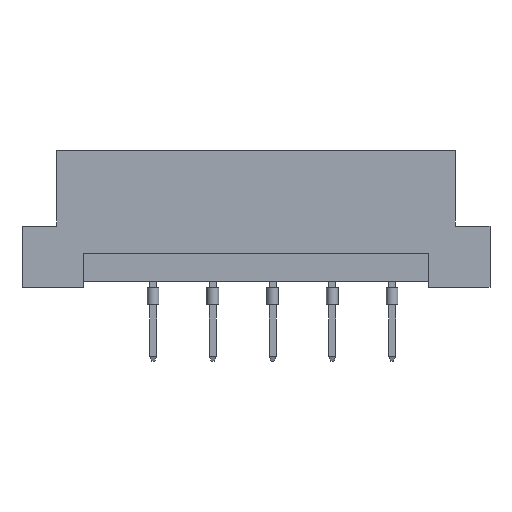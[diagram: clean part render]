
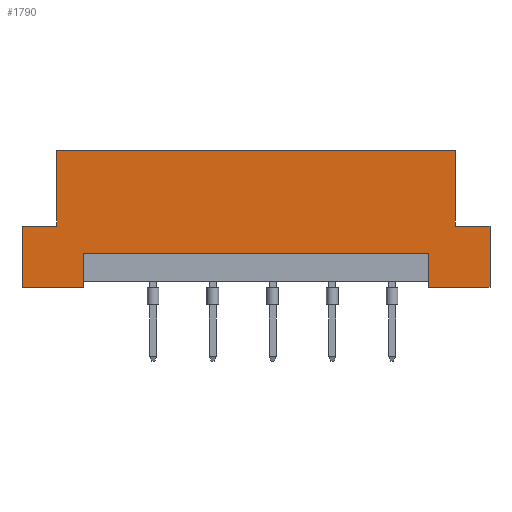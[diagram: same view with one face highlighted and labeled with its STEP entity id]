
A CAD part, front view. The second image highlights one B-rep face of the part: STEP entity #1790.
In plain terms, the highlighted planar face has unit normal (0, -1, 0).
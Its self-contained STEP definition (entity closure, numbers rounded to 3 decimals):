
#27 = CARTESIAN_POINT ( 'NONE',  ( -19.9, 0., 0. ) ) ;
#68 = LINE ( 'NONE', #2742, #5200 ) ;
#84 = CARTESIAN_POINT ( 'NONE',  ( -19.9, 0., 0. ) ) ;
#113 = LINE ( 'NONE', #6274, #5737 ) ;
#240 = VECTOR ( 'NONE', #1195, 1000. ) ;
#300 = VECTOR ( 'NONE', #1503, 1000. ) ;
#323 = ORIENTED_EDGE ( 'NONE', *, *, #650, .F. ) ;
#354 = DIRECTION ( 'NONE',  ( 0., 0., 1. ) ) ;
#372 = DIRECTION ( 'NONE',  ( 1., 0., 0. ) ) ;
#427 = ORIENTED_EDGE ( 'NONE', *, *, #1605, .F. ) ;
#447 = LINE ( 'NONE', #6684, #300 ) ;
#557 = DIRECTION ( 'NONE',  ( 1., 0., 0. ) ) ;
#596 = DIRECTION ( 'NONE',  ( 0., 0., -1. ) ) ;
#650 = EDGE_CURVE ( 'NONE', #3738, #4170, #4349, .T. ) ;
#774 = CARTESIAN_POINT ( 'NONE',  ( -16.94, 0., 5.2 ) ) ;
#821 = EDGE_CURVE ( 'NONE', #1131, #5283, #1346, .T. ) ;
#930 = CARTESIAN_POINT ( 'NONE',  ( 19.9, 0., 0. ) ) ;
#932 = CARTESIAN_POINT ( 'NONE',  ( -14.69, 0., 0. ) ) ;
#944 = CARTESIAN_POINT ( 'NONE',  ( 16.94, 0., 11.6 ) ) ;
#1004 = VERTEX_POINT ( 'NONE', #930 ) ;
#1118 = EDGE_CURVE ( 'NONE', #2424, #4580, #1618, .T. ) ;
#1131 = VERTEX_POINT ( 'NONE', #5353 ) ;
#1138 = EDGE_CURVE ( 'NONE', #5283, #4580, #113, .T. ) ;
#1169 = VECTOR ( 'NONE', #4728, 1000. ) ;
#1195 = DIRECTION ( 'NONE',  ( 0., 0., -1. ) ) ;
#1198 = VERTEX_POINT ( 'NONE', #2931 ) ;
#1230 = LINE ( 'NONE', #4291, #240 ) ;
#1299 = DIRECTION ( 'NONE',  ( 0., 0., 1. ) ) ;
#1346 = LINE ( 'NONE', #774, #3846 ) ;
#1361 = LINE ( 'NONE', #5511, #3336 ) ;
#1373 = VERTEX_POINT ( 'NONE', #1498 ) ;
#1493 = VECTOR ( 'NONE', #1299, 1000. ) ;
#1498 = CARTESIAN_POINT ( 'NONE',  ( 14.69, 0., 2.9 ) ) ;
#1503 = DIRECTION ( 'NONE',  ( -1., 0., 0. ) ) ;
#1559 = ORIENTED_EDGE ( 'NONE', *, *, #1784, .F. ) ;
#1605 = EDGE_CURVE ( 'NONE', #4170, #4579, #4368, .T. ) ;
#1618 = LINE ( 'NONE', #1654, #5959 ) ;
#1622 = LINE ( 'NONE', #5387, #6400 ) ;
#1654 = CARTESIAN_POINT ( 'NONE',  ( 16.94, 0., 5.2 ) ) ;
#1709 = ORIENTED_EDGE ( 'NONE', *, *, #3862, .T. ) ;
#1728 = CARTESIAN_POINT ( 'NONE',  ( -16.94, 0., 11.6 ) ) ;
#1729 = EDGE_CURVE ( 'NONE', #2424, #1198, #1361, .T. ) ;
#1784 = EDGE_CURVE ( 'NONE', #1198, #1004, #3977, .T. ) ;
#1790 = ADVANCED_FACE ( 'NONE', ( #2953 ), #4045, .F. ) ;
#2059 = EDGE_LOOP ( 'NONE', ( #2166, #1709, #3036, #1559, #6204, #4884, #3161, #4533, #6317, #427, #323, #4740 ) ) ;
#2166 = ORIENTED_EDGE ( 'NONE', *, *, #5589, .F. ) ;
#2204 = DIRECTION ( 'NONE',  ( 1., 0., 0. ) ) ;
#2424 = VERTEX_POINT ( 'NONE', #6031 ) ;
#2653 = LINE ( 'NONE', #3076, #1169 ) ;
#2742 = CARTESIAN_POINT ( 'NONE',  ( -19.9, 0., 5.2 ) ) ;
#2870 = VERTEX_POINT ( 'NONE', #3594 ) ;
#2931 = CARTESIAN_POINT ( 'NONE',  ( 19.9, 0., 5.2 ) ) ;
#2953 = FACE_OUTER_BOUND ( 'NONE', #2059, .T. ) ;
#2981 = CARTESIAN_POINT ( 'NONE',  ( -19.9, 0., 11.6 ) ) ;
#3013 = EDGE_CURVE ( 'NONE', #2870, #3738, #1230, .T. ) ;
#3036 = ORIENTED_EDGE ( 'NONE', *, *, #4673, .F. ) ;
#3076 = CARTESIAN_POINT ( 'NONE',  ( -19.9, 0., 0. ) ) ;
#3161 = ORIENTED_EDGE ( 'NONE', *, *, #1138, .F. ) ;
#3336 = VECTOR ( 'NONE', #372, 1000. ) ;
#3463 = CARTESIAN_POINT ( 'NONE',  ( -19.9, 0., 5.2 ) ) ;
#3494 = DIRECTION ( 'NONE',  ( 0., 0., -1. ) ) ;
#3594 = CARTESIAN_POINT ( 'NONE',  ( -14.69, 0., 2.9 ) ) ;
#3660 = AXIS2_PLACEMENT_3D ( 'NONE', #2981, #4500, #6120 ) ;
#3738 = VERTEX_POINT ( 'NONE', #932 ) ;
#3751 = DIRECTION ( 'NONE',  ( 0., 0., 1. ) ) ;
#3846 = VECTOR ( 'NONE', #354, 1000. ) ;
#3862 = EDGE_CURVE ( 'NONE', #1373, #5313, #1622, .T. ) ;
#3977 = LINE ( 'NONE', #5002, #6389 ) ;
#4045 = PLANE ( 'NONE',  #3660 ) ;
#4170 = VERTEX_POINT ( 'NONE', #27 ) ;
#4291 = CARTESIAN_POINT ( 'NONE',  ( -14.69, 0., 0.5 ) ) ;
#4349 = LINE ( 'NONE', #84, #5578 ) ;
#4368 = LINE ( 'NONE', #5410, #1493 ) ;
#4500 = DIRECTION ( 'NONE',  ( 0., 1., 0. ) ) ;
#4533 = ORIENTED_EDGE ( 'NONE', *, *, #821, .F. ) ;
#4579 = VERTEX_POINT ( 'NONE', #3463 ) ;
#4580 = VERTEX_POINT ( 'NONE', #944 ) ;
#4673 = EDGE_CURVE ( 'NONE', #1004, #5313, #2653, .T. ) ;
#4728 = DIRECTION ( 'NONE',  ( -1., 0., 0. ) ) ;
#4740 = ORIENTED_EDGE ( 'NONE', *, *, #3013, .F. ) ;
#4884 = ORIENTED_EDGE ( 'NONE', *, *, #1118, .T. ) ;
#5002 = CARTESIAN_POINT ( 'NONE',  ( 19.9, 0., 0. ) ) ;
#5200 = VECTOR ( 'NONE', #557, 1000. ) ;
#5228 = DIRECTION ( 'NONE',  ( -1., 0., 0. ) ) ;
#5283 = VERTEX_POINT ( 'NONE', #1728 ) ;
#5313 = VERTEX_POINT ( 'NONE', #6518 ) ;
#5353 = CARTESIAN_POINT ( 'NONE',  ( -16.94, 0., 5.2 ) ) ;
#5387 = CARTESIAN_POINT ( 'NONE',  ( 14.69, 0., 0.5 ) ) ;
#5410 = CARTESIAN_POINT ( 'NONE',  ( -19.9, 0., 0. ) ) ;
#5511 = CARTESIAN_POINT ( 'NONE',  ( 19.9, 0., 5.2 ) ) ;
#5578 = VECTOR ( 'NONE', #5228, 1000. ) ;
#5589 = EDGE_CURVE ( 'NONE', #1373, #2870, #447, .T. ) ;
#5737 = VECTOR ( 'NONE', #2204, 1000. ) ;
#5959 = VECTOR ( 'NONE', #3751, 1000. ) ;
#6031 = CARTESIAN_POINT ( 'NONE',  ( 16.94, 0., 5.2 ) ) ;
#6120 = DIRECTION ( 'NONE',  ( 0., 0., 1. ) ) ;
#6204 = ORIENTED_EDGE ( 'NONE', *, *, #1729, .F. ) ;
#6274 = CARTESIAN_POINT ( 'NONE',  ( -19.9, 0., 11.6 ) ) ;
#6317 = ORIENTED_EDGE ( 'NONE', *, *, #6543, .F. ) ;
#6389 = VECTOR ( 'NONE', #3494, 1000. ) ;
#6400 = VECTOR ( 'NONE', #596, 1000. ) ;
#6518 = CARTESIAN_POINT ( 'NONE',  ( 14.69, 0., 0. ) ) ;
#6543 = EDGE_CURVE ( 'NONE', #4579, #1131, #68, .T. ) ;
#6684 = CARTESIAN_POINT ( 'NONE',  ( 14.69, 0., 2.9 ) ) ;
